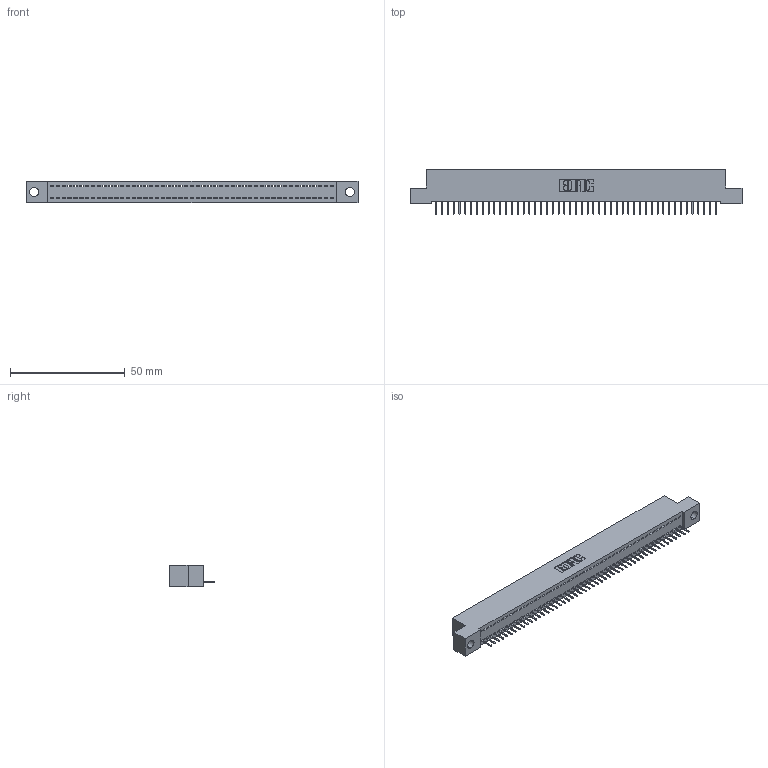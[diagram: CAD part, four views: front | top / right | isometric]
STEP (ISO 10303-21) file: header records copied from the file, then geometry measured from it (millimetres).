
FILE_DESCRIPTION (( 'STEP AP203' ), '1' );
FILE_NAME ('392-049-524-104.STEP', '2018-08-17T00:05:21', ( '' ), ( '' ), 'SwSTEP 2.0', 'SolidWorks 2016', '' );
FILE_SCHEMA (( 'CONFIG_CONTROL_DESIGN' ));
Length unit declared in the file: inch
Products named in the file (3): 342 Part_.156 TH; 345-292-001_345-293-124; 392-049-524-104
Assembly tree (50 placements, depth 2):
  392-049-524-104
    342 Part_.156 TH
    345-292-001_345-293-124  x49
Bounding box: 144.78 x 19.69 x 9.4 mm (x, y, z)
Volume: 12439.5 mm3; surface area: 17615.1 mm2
Topology: 50 solids, 50 shells, 3148 faces, 9119 edges, 5882 vertices
Faces by surface type: plane 2418, cylinder 730
Entity records: 28995 total; most frequent: CARTESIAN_POINT 5005, ORIENTED_EDGE 4990, DIRECTION 4209, EDGE_CURVE 2495, LINE 2371, VECTOR 2371, VERTEX_POINT 1658, AXIS2_PLACEMENT_3D 919
